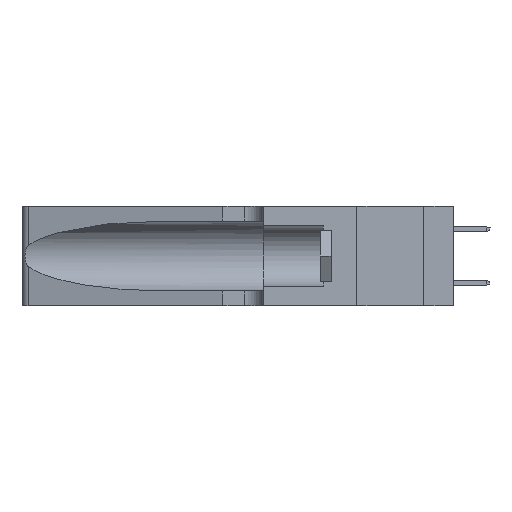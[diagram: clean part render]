
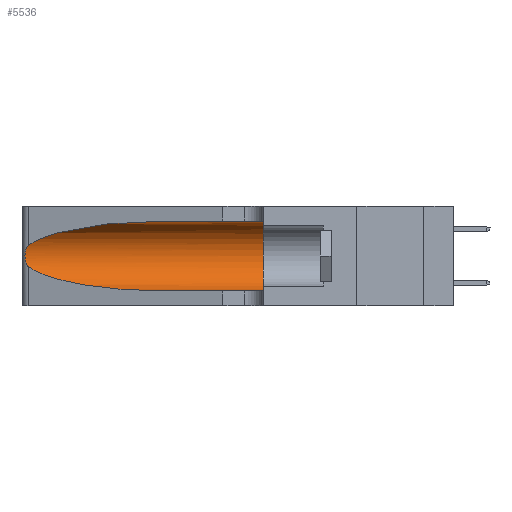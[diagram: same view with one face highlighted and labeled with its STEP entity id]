
A CAD part, left-side view. The second image highlights one B-rep face of the part: STEP entity #5536.
In plain terms, the highlighted cylindrical face has radius 3.308 mm (diameter 6.617 mm), a partial arc.
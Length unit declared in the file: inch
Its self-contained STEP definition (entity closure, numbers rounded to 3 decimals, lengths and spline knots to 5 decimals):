
#189 = VECTOR ( 'NONE', #4471, 39.37008 ) ;
#248 = CARTESIAN_POINT ( 'NONE',  ( 0.1305, 0.72297, 0.31525 ) ) ;
#784 = ORIENTED_EDGE ( 'NONE', *, *, #9256, .T. ) ;
#811 = EDGE_CURVE ( 'NONE', #17924, #11869, #2451, .T. ) ;
#1324 = DIRECTION ( 'NONE',  ( 0., 0., -1. ) ) ;
#1568 = CARTESIAN_POINT ( 'NONE',  ( 0.1305, 0.35, 0.05475 ) ) ;
#1629 = LINE ( 'NONE', #15929, #13924 ) ;
#1716 = VERTEX_POINT ( 'NONE', #17474 ) ;
#2223 = VERTEX_POINT ( 'NONE', #7500 ) ;
#2451 = CIRCLE ( 'NONE', #5172, 0.13025 ) ;
#2520 = VERTEX_POINT ( 'NONE', #20494 ) ;
#2548 = CARTESIAN_POINT ( 'NONE',  ( 0.1305, 0.72297, 0.05475 ) ) ;
#2799 = ORIENTED_EDGE ( 'NONE', *, *, #9711, .T. ) ;
#2999 = DIRECTION ( 'NONE',  ( 0., -1., 0. ) ) ;
#3407 = CARTESIAN_POINT ( 'NONE',  ( 0.25487, 1.22718, 0.14631 ) ) ;
#3749 = CARTESIAN_POINT ( 'NONE',  ( 0.25555, 1.22993, 0.14849 ) ) ;
#4171 = ORIENTED_EDGE ( 'NONE', *, *, #8954, .T. ) ;
#4335 = CARTESIAN_POINT ( 'NONE',  ( 0.25487, 1.22718, 0.22369 ) ) ;
#4471 = DIRECTION ( 'NONE',  ( 0., -1., 0. ) ) ;
#4514 = CARTESIAN_POINT ( 'NONE',  ( 0.25639, 1.23184, 0.21858 ) ) ;
#4616 = DIRECTION ( 'NONE',  ( 0., 0., 1. ) ) ;
#4931 = CARTESIAN_POINT ( 'NONE',  ( 0.25787, 1.23484, 0.2124 ) ) ;
#5024 = CARTESIAN_POINT ( 'NONE',  ( 0.2373, 1.15595, 0.28018 ) ) ;
#5172 = AXIS2_PLACEMENT_3D ( 'NONE', #14226, #12631, #4616 ) ;
#5536 = ADVANCED_FACE ( 'NONE', ( #11009 ), #9733, .F. ) ;
#5861 = EDGE_CURVE ( 'NONE', #1716, #17924, #9471, .T. ) ;
#6915 = CARTESIAN_POINT ( 'NONE',  ( 0.18966, 0.96281, 0.31525 ) ) ;
#7500 = CARTESIAN_POINT ( 'NONE',  ( 0.25487, 1.22718, 0.14631 ) ) ;
#7798 = CARTESIAN_POINT ( 'NONE',  ( 0.26075, 1.23896, 0.178 ) ) ;
#7896 = EDGE_CURVE ( 'NONE', #2520, #11869, #1629, .T. ) ;
#8113 = CARTESIAN_POINT ( 'NONE',  ( 0.1305, 1.61858, 0.185 ) ) ;
#8210 = ORIENTED_EDGE ( 'NONE', *, *, #7896, .T. ) ;
#8321 = AXIS2_PLACEMENT_3D ( 'NONE', #8113, #14651, #1324 ) ;
#8336 = CARTESIAN_POINT ( 'NONE',  ( 0.25639, 1.23186, 0.15144 ) ) ;
#8645 = CARTESIAN_POINT ( 'NONE',  ( 0.1305, 0.35, 0.31525 ) ) ;
#8954 = EDGE_CURVE ( 'NONE', #20247, #2223, #12401, .T. ) ;
#9256 = EDGE_CURVE ( 'NONE', #1716, #20247, #15963, .T. ) ;
#9471 = LINE ( 'NONE', #12719, #189 ) ;
#9711 = EDGE_CURVE ( 'NONE', #2223, #2520, #18129, .T. ) ;
#9733 = CYLINDRICAL_SURFACE ( 'NONE', #8321, 0.13025 ) ;
#9888 = CARTESIAN_POINT ( 'NONE',  ( 0.2373, 1.15595, 0.08982 ) ) ;
#10056 = CARTESIAN_POINT ( 'NONE',  ( 0.25487, 1.22718, 0.14631 ) ) ;
#11009 = FACE_OUTER_BOUND ( 'NONE', #12759, .T. ) ;
#11020 = CARTESIAN_POINT ( 'NONE',  ( 0.26018, 1.23835, 0.19895 ) ) ;
#11459 = CARTESIAN_POINT ( 'NONE',  ( 0.25854, 1.2359, 0.20912 ) ) ;
#11869 = VERTEX_POINT ( 'NONE', #1568 ) ;
#12401 = B_SPLINE_CURVE_WITH_KNOTS ( 'NONE', 3,
 ( #13069, #19553, #4514, #4931, #11459, #11020, #17548, #7798, #18377, #16377, #13389, #8336, #3749, #10056 ),
 .UNSPECIFIED., .F., .F.,
 ( 4, 2, 2, 2, 2, 2, 4 ),
 ( 0., 0.00027, 0.00053, 0.00107, 0.0016, 0.00187, 0.00214 ),
 .UNSPECIFIED. ) ;
#12631 = DIRECTION ( 'NONE',  ( 0., 1., 0. ) ) ;
#12719 = CARTESIAN_POINT ( 'NONE',  ( 0.1305, 1.61858, 0.31525 ) ) ;
#12759 = EDGE_LOOP ( 'NONE', ( #784, #4171, #2799, #8210, #20036, #20638 ) ) ;
#13069 = CARTESIAN_POINT ( 'NONE',  ( 0.25487, 1.22718, 0.22369 ) ) ;
#13389 = CARTESIAN_POINT ( 'NONE',  ( 0.25789, 1.23486, 0.15765 ) ) ;
#13924 = VECTOR ( 'NONE', #2999, 39.37008 ) ;
#14226 = CARTESIAN_POINT ( 'NONE',  ( 0.1305, 0.35, 0.185 ) ) ;
#14651 = DIRECTION ( 'NONE',  ( 0., -1., 0. ) ) ;
#15929 = CARTESIAN_POINT ( 'NONE',  ( 0.1305, 1.61858, 0.05475 ) ) ;
#15963 =( BOUNDED_CURVE ( )  B_SPLINE_CURVE ( 3, ( #248, #6915, #5024, #19948 ),
 .UNSPECIFIED., .F., .T. ) 
 B_SPLINE_CURVE_WITH_KNOTS ( ( 4, 4 ),
 ( 1.5708, 2.84003 ),
 .UNSPECIFIED. ) 
 CURVE ( )  GEOMETRIC_REPRESENTATION_ITEM ( )  RATIONAL_B_SPLINE_CURVE ( ( 1., 0.87, 0.87, 1. ) ) 
 REPRESENTATION_ITEM ( '' )  );
#16377 = CARTESIAN_POINT ( 'NONE',  ( 0.25856, 1.23593, 0.16098 ) ) ;
#16433 = CARTESIAN_POINT ( 'NONE',  ( 0.18966, 0.96281, 0.05475 ) ) ;
#17474 = CARTESIAN_POINT ( 'NONE',  ( 0.1305, 0.72297, 0.31525 ) ) ;
#17548 = CARTESIAN_POINT ( 'NONE',  ( 0.26075, 1.23896, 0.19203 ) ) ;
#17924 = VERTEX_POINT ( 'NONE', #8645 ) ;
#18129 =( BOUNDED_CURVE ( )  B_SPLINE_CURVE ( 3, ( #3407, #9888, #16433, #2548 ),
 .UNSPECIFIED., .F., .T. ) 
 B_SPLINE_CURVE_WITH_KNOTS ( ( 4, 4 ),
 ( 3.44316, 4.71239 ),
 .UNSPECIFIED. ) 
 CURVE ( )  GEOMETRIC_REPRESENTATION_ITEM ( )  RATIONAL_B_SPLINE_CURVE ( ( 1., 0.87, 0.87, 1. ) ) 
 REPRESENTATION_ITEM ( '' )  );
#18377 = CARTESIAN_POINT ( 'NONE',  ( 0.26017, 1.23833, 0.17102 ) ) ;
#19553 = CARTESIAN_POINT ( 'NONE',  ( 0.25555, 1.22994, 0.2215 ) ) ;
#19948 = CARTESIAN_POINT ( 'NONE',  ( 0.25487, 1.22718, 0.22369 ) ) ;
#20036 = ORIENTED_EDGE ( 'NONE', *, *, #811, .F. ) ;
#20247 = VERTEX_POINT ( 'NONE', #4335 ) ;
#20494 = CARTESIAN_POINT ( 'NONE',  ( 0.1305, 0.72297, 0.05475 ) ) ;
#20638 = ORIENTED_EDGE ( 'NONE', *, *, #5861, .F. ) ;
